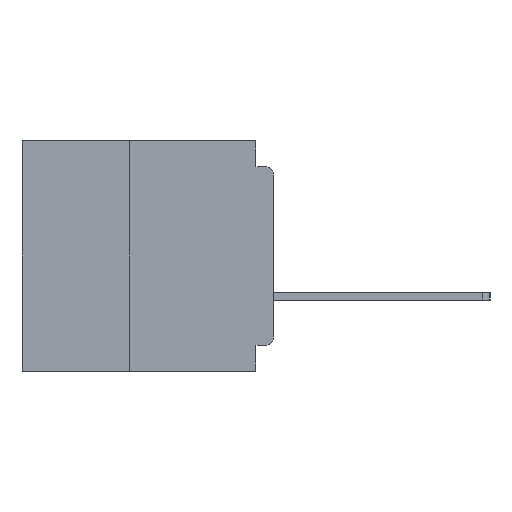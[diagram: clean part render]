
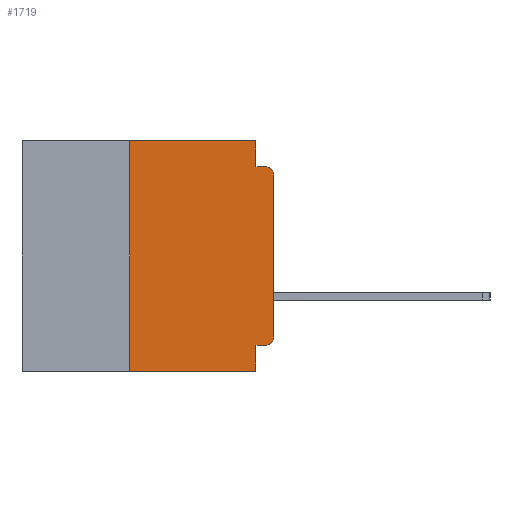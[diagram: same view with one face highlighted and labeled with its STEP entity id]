
A CAD part, left-side view. The second image highlights one B-rep face of the part: STEP entity #1719.
In plain terms, the highlighted planar face has unit normal (-1, 0, 0).
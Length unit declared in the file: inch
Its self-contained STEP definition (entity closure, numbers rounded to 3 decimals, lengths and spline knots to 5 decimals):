
#1080 = VERTEX_POINT ( 'NONE', #17237 ) ;
#1187 = ORIENTED_EDGE ( 'NONE', *, *, #24410, .F. ) ;
#1351 = DIRECTION ( 'NONE',  ( 0., -1., 0. ) ) ;
#1719 = ADVANCED_FACE ( 'NONE', ( #24260 ), #29680, .F. ) ;
#1838 = VERTEX_POINT ( 'NONE', #11581 ) ;
#2784 = VERTEX_POINT ( 'NONE', #22053 ) ;
#2789 = ORIENTED_EDGE ( 'NONE', *, *, #21052, .F. ) ;
#4098 = CARTESIAN_POINT ( 'NONE',  ( 0., 0.015, -0.34 ) ) ;
#4947 = LINE ( 'NONE', #7536, #33114 ) ;
#5744 = ORIENTED_EDGE ( 'NONE', *, *, #26797, .T. ) ;
#6344 = LINE ( 'NONE', #27210, #30234 ) ;
#6682 = LINE ( 'NONE', #8040, #38554 ) ;
#7254 = DIRECTION ( 'NONE',  ( 0., 0., -1. ) ) ;
#7536 = CARTESIAN_POINT ( 'NONE',  ( 0., 0., -0.355 ) ) ;
#8040 = CARTESIAN_POINT ( 'NONE',  ( 0., 0., 0. ) ) ;
#8239 = ORIENTED_EDGE ( 'NONE', *, *, #16876, .T. ) ;
#9376 = DIRECTION ( 'NONE',  ( -1., 0., 0. ) ) ;
#9423 = DIRECTION ( 'NONE',  ( 0., -1., 0. ) ) ;
#10335 = LINE ( 'NONE', #38494, #24018 ) ;
#10401 = VERTEX_POINT ( 'NONE', #24228 ) ;
#10787 = ORIENTED_EDGE ( 'NONE', *, *, #36086, .T. ) ;
#11047 = CARTESIAN_POINT ( 'NONE',  ( 0., 0.437, 0. ) ) ;
#11321 = CARTESIAN_POINT ( 'NONE',  ( 0., 0.25, 0. ) ) ;
#11376 = LINE ( 'NONE', #15819, #27038 ) ;
#11581 = CARTESIAN_POINT ( 'NONE',  ( 0., 0., -0.06 ) ) ;
#12476 = CIRCLE ( 'NONE', #31953, 0.015 ) ;
#13494 = VECTOR ( 'NONE', #16730, 39.37008 ) ;
#14195 = DIRECTION ( 'NONE',  ( 0., 0., -1. ) ) ;
#14604 = CARTESIAN_POINT ( 'NONE',  ( 0., 0.015, -0.045 ) ) ;
#15160 = EDGE_LOOP ( 'NONE', ( #10787, #17319, #18715, #1187, #32868, #2789, #8239, #24115, #17798, #5744 ) ) ;
#15819 = CARTESIAN_POINT ( 'NONE',  ( 0., 0.437, -0.4 ) ) ;
#16370 = CARTESIAN_POINT ( 'NONE',  ( 0., 0.031, -0.4 ) ) ;
#16730 = DIRECTION ( 'NONE',  ( 0., 0., -1. ) ) ;
#16876 = EDGE_CURVE ( 'NONE', #31286, #23128, #11376, .T. ) ;
#17000 = EDGE_CURVE ( 'NONE', #10401, #18089, #23112, .T. ) ;
#17077 = VERTEX_POINT ( 'NONE', #26246 ) ;
#17237 = CARTESIAN_POINT ( 'NONE',  ( 0., 0.015, -0.355 ) ) ;
#17319 = ORIENTED_EDGE ( 'NONE', *, *, #20040, .T. ) ;
#17798 = ORIENTED_EDGE ( 'NONE', *, *, #37808, .F. ) ;
#17919 = EDGE_CURVE ( 'NONE', #25693, #20829, #10335, .T. ) ;
#18089 = VERTEX_POINT ( 'NONE', #14604 ) ;
#18715 = ORIENTED_EDGE ( 'NONE', *, *, #17000, .F. ) ;
#20008 = CARTESIAN_POINT ( 'NONE',  ( 0., 0.031, 0. ) ) ;
#20040 = EDGE_CURVE ( 'NONE', #1838, #18089, #28909, .T. ) ;
#20658 = DIRECTION ( 'NONE',  ( 0., 0., 1. ) ) ;
#20829 = VERTEX_POINT ( 'NONE', #20008 ) ;
#21052 = EDGE_CURVE ( 'NONE', #31286, #25693, #6344, .T. ) ;
#22048 = DIRECTION ( 'NONE',  ( 0., 0., -1. ) ) ;
#22053 = CARTESIAN_POINT ( 'NONE',  ( 0., 0., -0.34 ) ) ;
#22339 = CARTESIAN_POINT ( 'NONE',  ( 0., 0.25, -0.4 ) ) ;
#23112 = LINE ( 'NONE', #31807, #38348 ) ;
#23128 = VERTEX_POINT ( 'NONE', #16370 ) ;
#24018 = VECTOR ( 'NONE', #1351, 39.37008 ) ;
#24115 = ORIENTED_EDGE ( 'NONE', *, *, #37516, .F. ) ;
#24228 = CARTESIAN_POINT ( 'NONE',  ( 0., 0.031, -0.045 ) ) ;
#24260 = FACE_OUTER_BOUND ( 'NONE', #15160, .T. ) ;
#24410 = EDGE_CURVE ( 'NONE', #20829, #10401, #37063, .T. ) ;
#25693 = VERTEX_POINT ( 'NONE', #11321 ) ;
#26031 = DIRECTION ( 'NONE',  ( -1., 0., 0. ) ) ;
#26205 = CARTESIAN_POINT ( 'NONE',  ( 0., 0.031, 0. ) ) ;
#26246 = CARTESIAN_POINT ( 'NONE',  ( 0., 0.031, -0.355 ) ) ;
#26797 = EDGE_CURVE ( 'NONE', #1080, #2784, #12476, .T. ) ;
#27038 = VECTOR ( 'NONE', #9423, 39.37008 ) ;
#27210 = CARTESIAN_POINT ( 'NONE',  ( 0., 0.25, -0.4 ) ) ;
#27438 = AXIS2_PLACEMENT_3D ( 'NONE', #11047, #32705, #14195 ) ;
#28088 = CARTESIAN_POINT ( 'NONE',  ( 0., 0.015, -0.06 ) ) ;
#28301 = CARTESIAN_POINT ( 'NONE',  ( 0., 0.031, -0.4 ) ) ;
#28909 = CIRCLE ( 'NONE', #34505, 0.015 ) ;
#29484 = DIRECTION ( 'NONE',  ( 0., 1., 0. ) ) ;
#29680 = PLANE ( 'NONE',  #27438 ) ;
#30234 = VECTOR ( 'NONE', #30242, 39.37008 ) ;
#30242 = DIRECTION ( 'NONE',  ( 0., 0., 1. ) ) ;
#30339 = VECTOR ( 'NONE', #22048, 39.37008 ) ;
#31122 = DIRECTION ( 'NONE',  ( 0., 0., -1. ) ) ;
#31286 = VERTEX_POINT ( 'NONE', #22339 ) ;
#31807 = CARTESIAN_POINT ( 'NONE',  ( 0., 0., -0.045 ) ) ;
#31943 = DIRECTION ( 'NONE',  ( 0., -1., 0. ) ) ;
#31953 = AXIS2_PLACEMENT_3D ( 'NONE', #4098, #26031, #7254 ) ;
#32705 = DIRECTION ( 'NONE',  ( 1., 0., 0. ) ) ;
#32868 = ORIENTED_EDGE ( 'NONE', *, *, #17919, .F. ) ;
#33114 = VECTOR ( 'NONE', #29484, 39.37008 ) ;
#34505 = AXIS2_PLACEMENT_3D ( 'NONE', #28088, #9376, #31122 ) ;
#36086 = EDGE_CURVE ( 'NONE', #2784, #1838, #6682, .T. ) ;
#37063 = LINE ( 'NONE', #26205, #13494 ) ;
#37516 = EDGE_CURVE ( 'NONE', #17077, #23128, #38353, .T. ) ;
#37808 = EDGE_CURVE ( 'NONE', #1080, #17077, #4947, .T. ) ;
#38348 = VECTOR ( 'NONE', #31943, 39.37008 ) ;
#38353 = LINE ( 'NONE', #28301, #30339 ) ;
#38494 = CARTESIAN_POINT ( 'NONE',  ( 0., 0.437, 0. ) ) ;
#38554 = VECTOR ( 'NONE', #20658, 39.37008 ) ;
